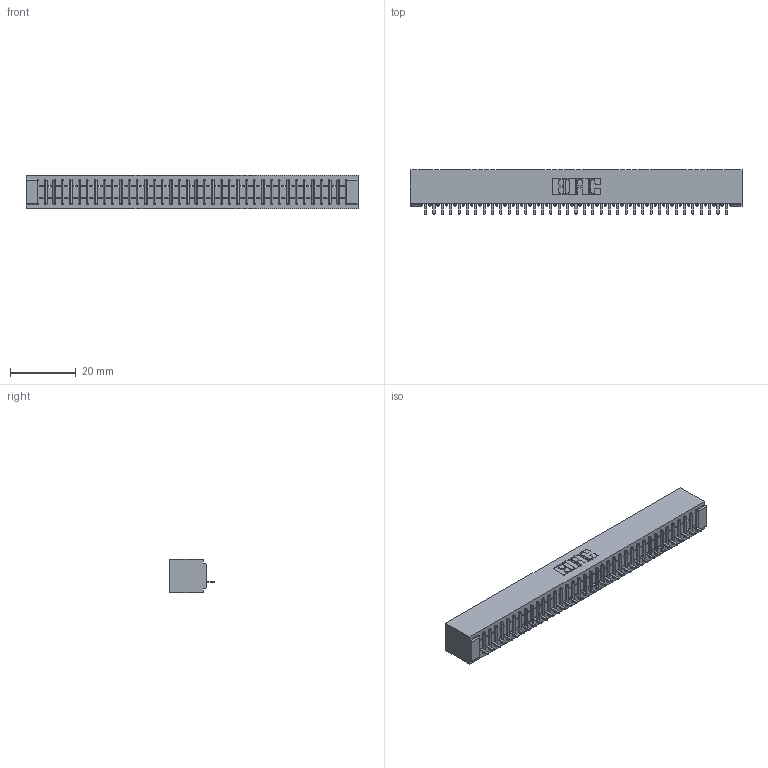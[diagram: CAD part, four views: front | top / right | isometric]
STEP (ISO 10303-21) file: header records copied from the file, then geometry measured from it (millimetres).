
FILE_DESCRIPTION (( 'STEP AP203' ), '1' );
FILE_NAME ('391-037-524-101.STEP', '2018-08-08T23:53:19', ( '' ), ( '' ), 'SwSTEP 2.0', 'SolidWorks 2016', '' );
FILE_SCHEMA (( 'CONFIG_CONTROL_DESIGN' ));
Length unit declared in the file: inch
Products named in the file (3): 341 Part_No Mounting Lugs; 341-292-001_341-292-124; 391-037-524-101
Assembly tree (38 placements, depth 2):
  391-037-524-101
    341 Part_No Mounting Lugs
    341-292-001_341-292-124  x37
Bounding box: 100.97 x 13.64 x 10.16 mm (x, y, z)
Volume: 7418.9 mm3; surface area: 11760.2 mm2
Topology: 38 solids, 38 shells, 3142 faces, 9061 edges, 5814 vertices
Faces by surface type: plane 1951, cylinder 1043, sphere 76, torus 72
Entity records: 43982 total; most frequent: CARTESIAN_POINT 7470, ORIENTED_EDGE 7458, DIRECTION 7213, EDGE_CURVE 3729, VECTOR 3011, LINE 3011, VERTEX_POINT 2358, AXIS2_PLACEMENT_3D 2101
